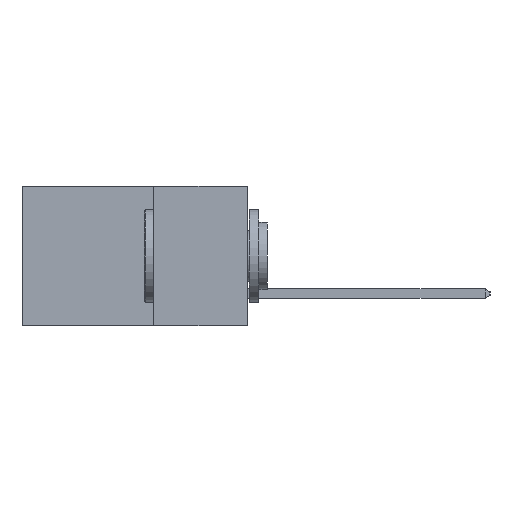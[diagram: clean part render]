
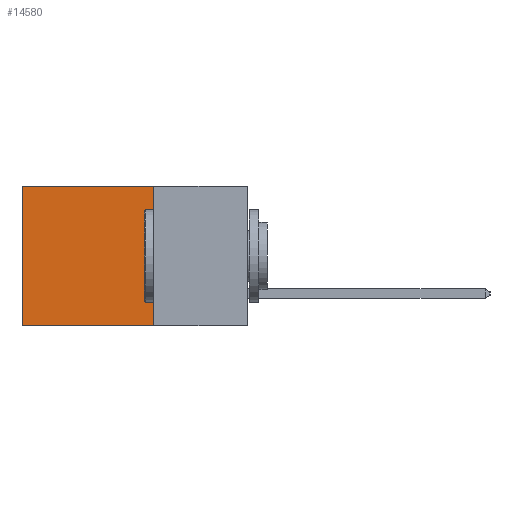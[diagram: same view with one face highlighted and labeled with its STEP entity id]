
A CAD part, left-side view. The second image highlights one B-rep face of the part: STEP entity #14580.
In plain terms, the highlighted planar face has unit normal (-1, 0, 0).
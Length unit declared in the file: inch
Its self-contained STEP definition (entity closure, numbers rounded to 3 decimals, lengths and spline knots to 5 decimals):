
#399 = AXIS2_PLACEMENT_3D ( 'NONE', #15939, #10206, #1277 ) ;
#614 = DIRECTION ( 'NONE',  ( 0., 1., 0. ) ) ;
#1277 = DIRECTION ( 'NONE',  ( 0., 0., -1. ) ) ;
#1652 = VECTOR ( 'NONE', #15699, 39.37008 ) ;
#2227 = VERTEX_POINT ( 'NONE', #7165 ) ;
#2253 = VECTOR ( 'NONE', #614, 39.37008 ) ;
#2906 = EDGE_CURVE ( 'NONE', #4095, #18633, #16539, .T. ) ;
#3566 = ORIENTED_EDGE ( 'NONE', *, *, #8100, .T. ) ;
#4095 = VERTEX_POINT ( 'NONE', #11944 ) ;
#5365 = VECTOR ( 'NONE', #17579, 39.37008 ) ;
#5696 = CARTESIAN_POINT ( 'NONE',  ( 0.298, 0.25, -0.37 ) ) ;
#6843 = EDGE_LOOP ( 'NONE', ( #7496, #11633, #10366, #3566 ) ) ;
#7165 = CARTESIAN_POINT ( 'NONE',  ( 0.298, 0.6, 0. ) ) ;
#7496 = ORIENTED_EDGE ( 'NONE', *, *, #8515, .T. ) ;
#7874 = DIRECTION ( 'NONE',  ( 0., 0., -1. ) ) ;
#8084 = CARTESIAN_POINT ( 'NONE',  ( 0.298, 0.25, -0.37 ) ) ;
#8100 = EDGE_CURVE ( 'NONE', #4095, #2227, #13475, .T. ) ;
#8380 = FACE_OUTER_BOUND ( 'NONE', #6843, .T. ) ;
#8476 = CARTESIAN_POINT ( 'NONE',  ( 0.298, 0.25, 0. ) ) ;
#8515 = EDGE_CURVE ( 'NONE', #2227, #14158, #18112, .T. ) ;
#10165 = LINE ( 'NONE', #8084, #2253 ) ;
#10206 = DIRECTION ( 'NONE',  ( 1., 0., 0. ) ) ;
#10366 = ORIENTED_EDGE ( 'NONE', *, *, #2906, .F. ) ;
#10466 = EDGE_CURVE ( 'NONE', #18633, #14158, #10165, .T. ) ;
#11633 = ORIENTED_EDGE ( 'NONE', *, *, #10466, .F. ) ;
#11944 = CARTESIAN_POINT ( 'NONE',  ( 0.298, 0.25, 0. ) ) ;
#12650 = CARTESIAN_POINT ( 'NONE',  ( 0.298, 0.25, 0. ) ) ;
#13475 = LINE ( 'NONE', #8476, #1652 ) ;
#14158 = VERTEX_POINT ( 'NONE', #16460 ) ;
#14514 = PLANE ( 'NONE',  #399 ) ;
#14580 = ADVANCED_FACE ( 'NONE', ( #8380 ), #14514, .F. ) ;
#15699 = DIRECTION ( 'NONE',  ( 0., 1., 0. ) ) ;
#15939 = CARTESIAN_POINT ( 'NONE',  ( 0.298, 0.25, 0. ) ) ;
#16460 = CARTESIAN_POINT ( 'NONE',  ( 0.298, 0.6, -0.37 ) ) ;
#16539 = LINE ( 'NONE', #12650, #5365 ) ;
#16560 = CARTESIAN_POINT ( 'NONE',  ( 0.298, 0.6, 0. ) ) ;
#17579 = DIRECTION ( 'NONE',  ( 0., 0., -1. ) ) ;
#17675 = VECTOR ( 'NONE', #7874, 39.37008 ) ;
#18112 = LINE ( 'NONE', #16560, #17675 ) ;
#18633 = VERTEX_POINT ( 'NONE', #5696 ) ;
